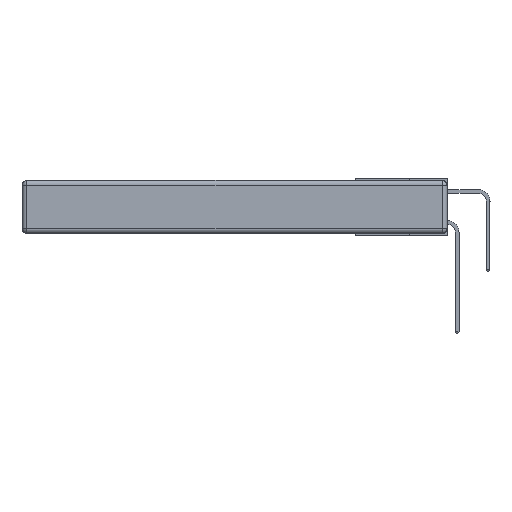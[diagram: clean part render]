
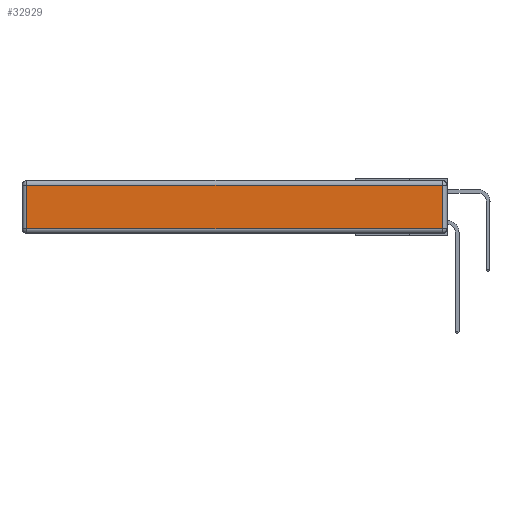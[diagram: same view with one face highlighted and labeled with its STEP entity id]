
A CAD part, left-side view. The second image highlights one B-rep face of the part: STEP entity #32929.
In plain terms, the highlighted planar face has unit normal (-1, 0, 0).
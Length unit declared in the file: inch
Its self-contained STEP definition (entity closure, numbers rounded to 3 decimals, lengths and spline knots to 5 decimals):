
#1113 = CARTESIAN_POINT ( 'NONE',  ( 0., 0.03, -0.03 ) ) ;
#2305 = EDGE_CURVE ( 'NONE', #27383, #8238, #5217, .T. ) ;
#2838 = DIRECTION ( 'NONE',  ( 0., 0., -1. ) ) ;
#2898 = CARTESIAN_POINT ( 'NONE',  ( 0., 0., -0.313 ) ) ;
#3107 = VECTOR ( 'NONE', #2838, 39.37008 ) ;
#5217 = LINE ( 'NONE', #30943, #11895 ) ;
#5593 = EDGE_LOOP ( 'NONE', ( #34511, #19433, #24521, #12238 ) ) ;
#6439 = VERTEX_POINT ( 'NONE', #29675 ) ;
#6944 = CARTESIAN_POINT ( 'NONE',  ( 0., 0.03, -0.313 ) ) ;
#8074 = PLANE ( 'NONE',  #34021 ) ;
#8238 = VERTEX_POINT ( 'NONE', #27905 ) ;
#8710 = CARTESIAN_POINT ( 'NONE',  ( 0., 2.72, -0.343 ) ) ;
#9610 = DIRECTION ( 'NONE',  ( 0., 0., 1. ) ) ;
#9636 = LINE ( 'NONE', #32274, #18081 ) ;
#10656 = EDGE_CURVE ( 'NONE', #6439, #16917, #16105, .T. ) ;
#10940 = DIRECTION ( 'NONE',  ( -1., 0., 0. ) ) ;
#11895 = VECTOR ( 'NONE', #19885, 39.37008 ) ;
#12238 = ORIENTED_EDGE ( 'NONE', *, *, #35512, .T. ) ;
#16105 = LINE ( 'NONE', #2898, #30473 ) ;
#16742 = DIRECTION ( 'NONE',  ( 0., -1., 0. ) ) ;
#16917 = VERTEX_POINT ( 'NONE', #6944 ) ;
#18081 = VECTOR ( 'NONE', #9610, 39.37008 ) ;
#18279 = LINE ( 'NONE', #8710, #3107 ) ;
#19433 = ORIENTED_EDGE ( 'NONE', *, *, #27863, .T. ) ;
#19885 = DIRECTION ( 'NONE',  ( 0., 1., 0. ) ) ;
#24521 = ORIENTED_EDGE ( 'NONE', *, *, #2305, .T. ) ;
#27383 = VERTEX_POINT ( 'NONE', #1113 ) ;
#27863 = EDGE_CURVE ( 'NONE', #16917, #27383, #9636, .T. ) ;
#27905 = CARTESIAN_POINT ( 'NONE',  ( 0., 2.72, -0.03 ) ) ;
#28099 = CARTESIAN_POINT ( 'NONE',  ( 0., 0., -0.343 ) ) ;
#29675 = CARTESIAN_POINT ( 'NONE',  ( 0., 2.72, -0.313 ) ) ;
#29700 = FACE_OUTER_BOUND ( 'NONE', #5593, .T. ) ;
#30473 = VECTOR ( 'NONE', #16742, 39.37008 ) ;
#30943 = CARTESIAN_POINT ( 'NONE',  ( 0., 2.75, -0.03 ) ) ;
#32274 = CARTESIAN_POINT ( 'NONE',  ( 0., 0.03, -0.343 ) ) ;
#32929 = ADVANCED_FACE ( 'NONE', ( #29700 ), #8074, .T. ) ;
#33874 = DIRECTION ( 'NONE',  ( 0., 0., 1. ) ) ;
#34021 = AXIS2_PLACEMENT_3D ( 'NONE', #28099, #10940, #33874 ) ;
#34511 = ORIENTED_EDGE ( 'NONE', *, *, #10656, .T. ) ;
#35512 = EDGE_CURVE ( 'NONE', #8238, #6439, #18279, .T. ) ;
